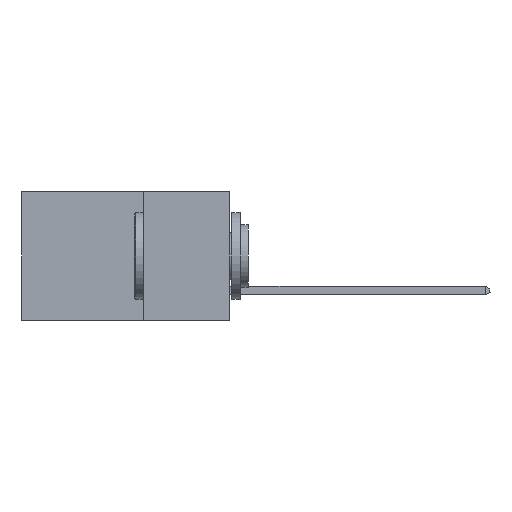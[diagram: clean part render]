
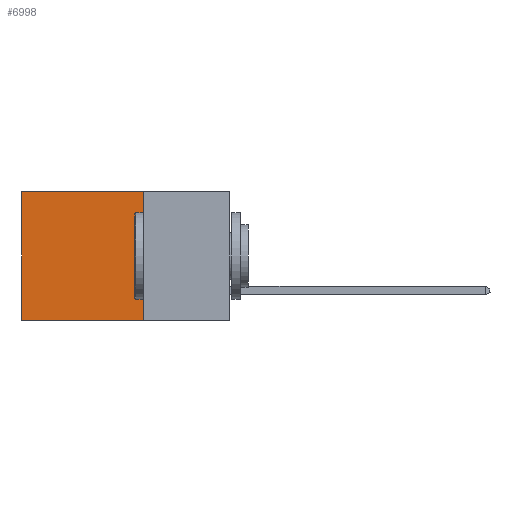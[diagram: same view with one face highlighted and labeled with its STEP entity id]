
A CAD part, left-side view. The second image highlights one B-rep face of the part: STEP entity #6998.
In plain terms, the highlighted planar face has unit normal (-1, 0, 0).
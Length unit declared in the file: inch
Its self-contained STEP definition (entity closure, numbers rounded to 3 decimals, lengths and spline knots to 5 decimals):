
#1180 = EDGE_CURVE ( 'NONE', #30307, #2597, #18301, .T. ) ;
#2597 = VERTEX_POINT ( 'NONE', #10104 ) ;
#3084 = EDGE_CURVE ( 'NONE', #15623, #2597, #27885, .T. ) ;
#3633 = ORIENTED_EDGE ( 'NONE', *, *, #18695, .F. ) ;
#4000 = CARTESIAN_POINT ( 'NONE',  ( 0.298, 0.6, 0. ) ) ;
#4099 = VERTEX_POINT ( 'NONE', #15884 ) ;
#4794 = VECTOR ( 'NONE', #27030, 39.37008 ) ;
#6986 = AXIS2_PLACEMENT_3D ( 'NONE', #8622, #29036, #11740 ) ;
#6998 = ADVANCED_FACE ( 'NONE', ( #10489 ), #11427, .F. ) ;
#8622 = CARTESIAN_POINT ( 'NONE',  ( 0.298, 0.25, 0. ) ) ;
#9925 = CARTESIAN_POINT ( 'NONE',  ( 0.298, 0.6, 0. ) ) ;
#10104 = CARTESIAN_POINT ( 'NONE',  ( 0.298, 0.6, -0.37 ) ) ;
#10489 = FACE_OUTER_BOUND ( 'NONE', #10907, .T. ) ;
#10799 = EDGE_CURVE ( 'NONE', #4099, #30307, #14900, .T. ) ;
#10907 = EDGE_LOOP ( 'NONE', ( #15047, #15846, #3633, #17195 ) ) ;
#11427 = PLANE ( 'NONE',  #6986 ) ;
#11740 = DIRECTION ( 'NONE',  ( 0., 0., -1. ) ) ;
#13550 = CARTESIAN_POINT ( 'NONE',  ( 0.298, 0.25, -0.37 ) ) ;
#14900 = LINE ( 'NONE', #24965, #4794 ) ;
#15047 = ORIENTED_EDGE ( 'NONE', *, *, #1180, .T. ) ;
#15599 = CARTESIAN_POINT ( 'NONE',  ( 0.298, 0.25, 0. ) ) ;
#15623 = VERTEX_POINT ( 'NONE', #13550 ) ;
#15846 = ORIENTED_EDGE ( 'NONE', *, *, #3084, .F. ) ;
#15884 = CARTESIAN_POINT ( 'NONE',  ( 0.298, 0.25, 0. ) ) ;
#17195 = ORIENTED_EDGE ( 'NONE', *, *, #10799, .T. ) ;
#17321 = DIRECTION ( 'NONE',  ( 0., 0., -1. ) ) ;
#17748 = VECTOR ( 'NONE', #28736, 39.37008 ) ;
#18301 = LINE ( 'NONE', #9925, #23415 ) ;
#18695 = EDGE_CURVE ( 'NONE', #4099, #15623, #20318, .T. ) ;
#20318 = LINE ( 'NONE', #15599, #28035 ) ;
#23415 = VECTOR ( 'NONE', #17321, 39.37008 ) ;
#23468 = CARTESIAN_POINT ( 'NONE',  ( 0.298, 0.25, -0.37 ) ) ;
#24965 = CARTESIAN_POINT ( 'NONE',  ( 0.298, 0.25, 0. ) ) ;
#27030 = DIRECTION ( 'NONE',  ( 0., 1., 0. ) ) ;
#27885 = LINE ( 'NONE', #23468, #17748 ) ;
#28025 = DIRECTION ( 'NONE',  ( 0., 0., -1. ) ) ;
#28035 = VECTOR ( 'NONE', #28025, 39.37008 ) ;
#28736 = DIRECTION ( 'NONE',  ( 0., 1., 0. ) ) ;
#29036 = DIRECTION ( 'NONE',  ( 1., 0., 0. ) ) ;
#30307 = VERTEX_POINT ( 'NONE', #4000 ) ;
